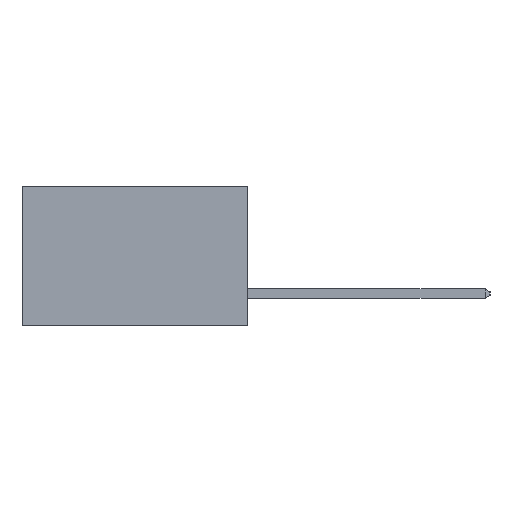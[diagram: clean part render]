
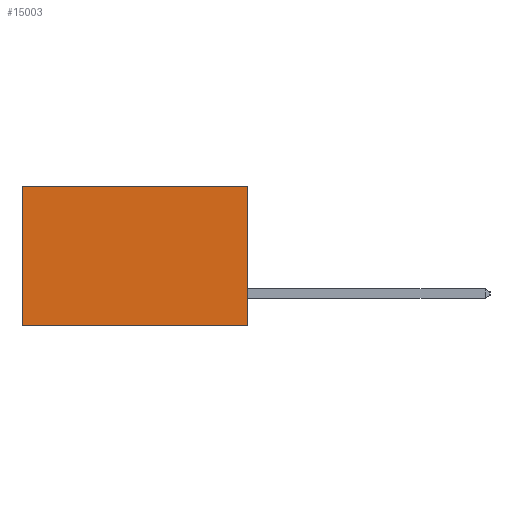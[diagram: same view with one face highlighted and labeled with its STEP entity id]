
A CAD part, left-side view. The second image highlights one B-rep face of the part: STEP entity #15003.
In plain terms, the highlighted planar face has unit normal (-1, 0, 0).
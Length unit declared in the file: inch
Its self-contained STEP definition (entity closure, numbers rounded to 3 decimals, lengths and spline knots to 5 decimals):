
#1235 = LINE ( 'NONE', #3132, #4780 ) ;
#1486 = VECTOR ( 'NONE', #5511, 39.37008 ) ;
#3000 = EDGE_CURVE ( 'NONE', #9365, #3579, #12035, .T. ) ;
#3008 = DIRECTION ( 'NONE',  ( 0., 1., 0. ) ) ;
#3132 = CARTESIAN_POINT ( 'NONE',  ( 0.2615, 0., 0. ) ) ;
#3456 = VERTEX_POINT ( 'NONE', #7915 ) ;
#3579 = VERTEX_POINT ( 'NONE', #4444 ) ;
#3732 = CARTESIAN_POINT ( 'NONE',  ( 0.2615, 0., -0.37 ) ) ;
#3917 = EDGE_LOOP ( 'NONE', ( #12827, #7819, #17627, #12193 ) ) ;
#4444 = CARTESIAN_POINT ( 'NONE',  ( 0.2615, 0.6, -0.37 ) ) ;
#4780 = VECTOR ( 'NONE', #3008, 39.37008 ) ;
#4911 = FACE_OUTER_BOUND ( 'NONE', #3917, .T. ) ;
#5186 = DIRECTION ( 'NONE',  ( 0., 0., -1. ) ) ;
#5511 = DIRECTION ( 'NONE',  ( 0., 0., -1. ) ) ;
#5698 = CARTESIAN_POINT ( 'NONE',  ( 0.2615, 0., -0.37 ) ) ;
#6749 = VECTOR ( 'NONE', #14386, 39.37008 ) ;
#7297 = CARTESIAN_POINT ( 'NONE',  ( 0.2615, 0., -0.37 ) ) ;
#7479 = CARTESIAN_POINT ( 'NONE',  ( 0.2615, 0.6, -0.37 ) ) ;
#7819 = ORIENTED_EDGE ( 'NONE', *, *, #3000, .F. ) ;
#7915 = CARTESIAN_POINT ( 'NONE',  ( 0.2615, 0., 0. ) ) ;
#8040 = DIRECTION ( 'NONE',  ( 0., 1., 0. ) ) ;
#9365 = VERTEX_POINT ( 'NONE', #13740 ) ;
#9529 = PLANE ( 'NONE',  #12861 ) ;
#10537 = EDGE_CURVE ( 'NONE', #3456, #9365, #16544, .T. ) ;
#10782 = EDGE_CURVE ( 'NONE', #3456, #17319, #1235, .T. ) ;
#12035 = LINE ( 'NONE', #7297, #14784 ) ;
#12193 = ORIENTED_EDGE ( 'NONE', *, *, #10782, .T. ) ;
#12220 = CARTESIAN_POINT ( 'NONE',  ( 0.2615, 0.6, 0. ) ) ;
#12827 = ORIENTED_EDGE ( 'NONE', *, *, #13212, .T. ) ;
#12861 = AXIS2_PLACEMENT_3D ( 'NONE', #3732, #13661, #5186 ) ;
#13212 = EDGE_CURVE ( 'NONE', #17319, #3579, #17586, .T. ) ;
#13661 = DIRECTION ( 'NONE',  ( 1., 0., 0. ) ) ;
#13740 = CARTESIAN_POINT ( 'NONE',  ( 0.2615, 0., -0.37 ) ) ;
#14386 = DIRECTION ( 'NONE',  ( 0., 0., -1. ) ) ;
#14784 = VECTOR ( 'NONE', #8040, 39.37008 ) ;
#15003 = ADVANCED_FACE ( 'NONE', ( #4911 ), #9529, .F. ) ;
#16544 = LINE ( 'NONE', #5698, #1486 ) ;
#17319 = VERTEX_POINT ( 'NONE', #12220 ) ;
#17586 = LINE ( 'NONE', #7479, #6749 ) ;
#17627 = ORIENTED_EDGE ( 'NONE', *, *, #10537, .F. ) ;
